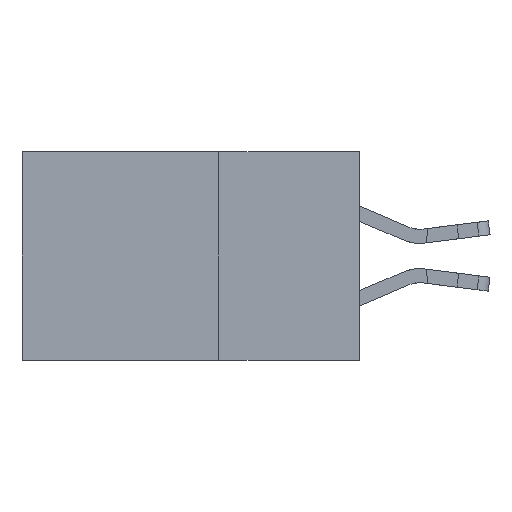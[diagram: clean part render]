
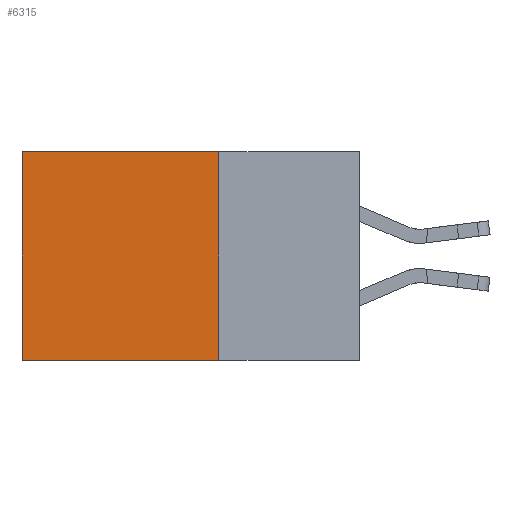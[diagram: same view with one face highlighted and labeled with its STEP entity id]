
A CAD part, left-side view. The second image highlights one B-rep face of the part: STEP entity #6315.
In plain terms, the highlighted planar face has unit normal (-1, 0, 0).
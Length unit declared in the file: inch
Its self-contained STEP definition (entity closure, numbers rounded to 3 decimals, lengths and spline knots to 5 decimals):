
#147 = CARTESIAN_POINT ( 'NONE',  ( 0.2875, 0.25, -0.37 ) ) ;
#319 = VECTOR ( 'NONE', #13744, 39.37008 ) ;
#510 = LINE ( 'NONE', #1323, #9389 ) ;
#554 = ORIENTED_EDGE ( 'NONE', *, *, #9176, .T. ) ;
#844 = CARTESIAN_POINT ( 'NONE',  ( 0.2875, 0.25, 0. ) ) ;
#1138 = EDGE_CURVE ( 'NONE', #12946, #7707, #11932, .T. ) ;
#1323 = CARTESIAN_POINT ( 'NONE',  ( 0.2875, 0.6, 0. ) ) ;
#1471 = CARTESIAN_POINT ( 'NONE',  ( 0.2875, 0.25, 0. ) ) ;
#1910 = CARTESIAN_POINT ( 'NONE',  ( 0.2875, 0.25, -0.37 ) ) ;
#2626 = LINE ( 'NONE', #18656, #21126 ) ;
#2665 = PLANE ( 'NONE',  #17953 ) ;
#5184 = EDGE_LOOP ( 'NONE', ( #11565, #10553, #21309, #554 ) ) ;
#5295 = LINE ( 'NONE', #844, #319 ) ;
#6315 = ADVANCED_FACE ( 'NONE', ( #15106 ), #2665, .F. ) ;
#7405 = CARTESIAN_POINT ( 'NONE',  ( 0.2875, 0.6, -0.37 ) ) ;
#7707 = VERTEX_POINT ( 'NONE', #7405 ) ;
#7832 = DIRECTION ( 'NONE',  ( 0., 0., -1. ) ) ;
#9176 = EDGE_CURVE ( 'NONE', #21111, #20357, #5295, .T. ) ;
#9389 = VECTOR ( 'NONE', #13037, 39.37008 ) ;
#10553 = ORIENTED_EDGE ( 'NONE', *, *, #1138, .F. ) ;
#11565 = ORIENTED_EDGE ( 'NONE', *, *, #17566, .T. ) ;
#11932 = LINE ( 'NONE', #147, #18733 ) ;
#12014 = DIRECTION ( 'NONE',  ( 0., 1., 0. ) ) ;
#12020 = CARTESIAN_POINT ( 'NONE',  ( 0.2875, 0.25, 0. ) ) ;
#12946 = VERTEX_POINT ( 'NONE', #1910 ) ;
#13037 = DIRECTION ( 'NONE',  ( 0., 0., -1. ) ) ;
#13176 = DIRECTION ( 'NONE',  ( 1., 0., 0. ) ) ;
#13744 = DIRECTION ( 'NONE',  ( 0., 1., 0. ) ) ;
#15106 = FACE_OUTER_BOUND ( 'NONE', #5184, .T. ) ;
#15192 = DIRECTION ( 'NONE',  ( 0., 0., -1. ) ) ;
#16453 = CARTESIAN_POINT ( 'NONE',  ( 0.2875, 0.6, 0. ) ) ;
#17566 = EDGE_CURVE ( 'NONE', #20357, #7707, #510, .T. ) ;
#17921 = EDGE_CURVE ( 'NONE', #21111, #12946, #2626, .T. ) ;
#17953 = AXIS2_PLACEMENT_3D ( 'NONE', #1471, #13176, #7832 ) ;
#18656 = CARTESIAN_POINT ( 'NONE',  ( 0.2875, 0.25, 0. ) ) ;
#18733 = VECTOR ( 'NONE', #12014, 39.37008 ) ;
#20357 = VERTEX_POINT ( 'NONE', #16453 ) ;
#21111 = VERTEX_POINT ( 'NONE', #12020 ) ;
#21126 = VECTOR ( 'NONE', #15192, 39.37008 ) ;
#21309 = ORIENTED_EDGE ( 'NONE', *, *, #17921, .F. ) ;
